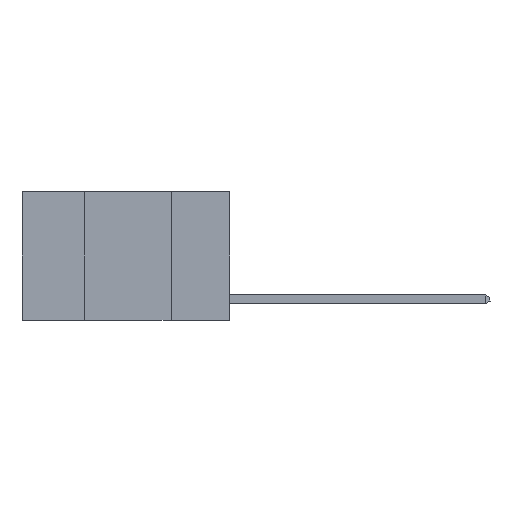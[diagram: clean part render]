
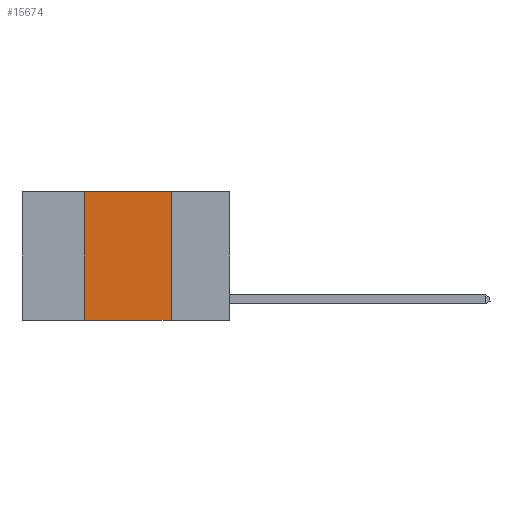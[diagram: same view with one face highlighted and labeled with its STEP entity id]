
A CAD part, left-side view. The second image highlights one B-rep face of the part: STEP entity #15674.
In plain terms, the highlighted planar face has unit normal (-1, 0, 0).
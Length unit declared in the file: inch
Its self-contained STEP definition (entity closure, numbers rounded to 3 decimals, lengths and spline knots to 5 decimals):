
#55 = EDGE_CURVE ( 'NONE', #5977, #15244, #16247, .T. ) ;
#549 = DIRECTION ( 'NONE',  ( 1., 0., 0. ) ) ;
#750 = FACE_OUTER_BOUND ( 'NONE', #3024, .T. ) ;
#1210 = ORIENTED_EDGE ( 'NONE', *, *, #18092, .F. ) ;
#1729 = VERTEX_POINT ( 'NONE', #17990 ) ;
#1797 = DIRECTION ( 'NONE',  ( 0., -1., 0. ) ) ;
#1864 = VECTOR ( 'NONE', #12312, 39.37008 ) ;
#1916 = ORIENTED_EDGE ( 'NONE', *, *, #20324, .F. ) ;
#3024 = EDGE_LOOP ( 'NONE', ( #1210, #1916, #11726, #22029 ) ) ;
#4125 = PLANE ( 'NONE',  #21698 ) ;
#5633 = LINE ( 'NONE', #10703, #19856 ) ;
#5977 = VERTEX_POINT ( 'NONE', #14188 ) ;
#6012 = LINE ( 'NONE', #17478, #1864 ) ;
#6310 = CARTESIAN_POINT ( 'NONE',  ( 0., 0.17, -0.37 ) ) ;
#7263 = DIRECTION ( 'NONE',  ( 0., 0., -1. ) ) ;
#9242 = CARTESIAN_POINT ( 'NONE',  ( 0., 0.6, 0. ) ) ;
#10291 = DIRECTION ( 'NONE',  ( 0., -1., 0. ) ) ;
#10703 = CARTESIAN_POINT ( 'NONE',  ( 0., 0.17, 0. ) ) ;
#11192 = VECTOR ( 'NONE', #10291, 39.37008 ) ;
#11726 = ORIENTED_EDGE ( 'NONE', *, *, #22985, .F. ) ;
#12312 = DIRECTION ( 'NONE',  ( 0., 0., 1. ) ) ;
#12738 = VECTOR ( 'NONE', #1797, 39.37008 ) ;
#13028 = LINE ( 'NONE', #19925, #12738 ) ;
#14188 = CARTESIAN_POINT ( 'NONE',  ( 0., 0.42, -0.37 ) ) ;
#15244 = VERTEX_POINT ( 'NONE', #6310 ) ;
#15674 = ADVANCED_FACE ( 'NONE', ( #750 ), #4125, .F. ) ;
#16247 = LINE ( 'NONE', #21051, #11192 ) ;
#17478 = CARTESIAN_POINT ( 'NONE',  ( 0., 0.42, 0. ) ) ;
#17990 = CARTESIAN_POINT ( 'NONE',  ( 0., 0.42, 0. ) ) ;
#18092 = EDGE_CURVE ( 'NONE', #20937, #15244, #5633, .T. ) ;
#19734 = DIRECTION ( 'NONE',  ( 0., 0., -1. ) ) ;
#19856 = VECTOR ( 'NONE', #19734, 39.37008 ) ;
#19925 = CARTESIAN_POINT ( 'NONE',  ( 0., 0.6, 0. ) ) ;
#20324 = EDGE_CURVE ( 'NONE', #1729, #20937, #13028, .T. ) ;
#20749 = CARTESIAN_POINT ( 'NONE',  ( 0., 0.17, 0. ) ) ;
#20937 = VERTEX_POINT ( 'NONE', #20749 ) ;
#21051 = CARTESIAN_POINT ( 'NONE',  ( 0., 0.6, -0.37 ) ) ;
#21698 = AXIS2_PLACEMENT_3D ( 'NONE', #9242, #549, #7263 ) ;
#22029 = ORIENTED_EDGE ( 'NONE', *, *, #55, .T. ) ;
#22985 = EDGE_CURVE ( 'NONE', #5977, #1729, #6012, .T. ) ;
